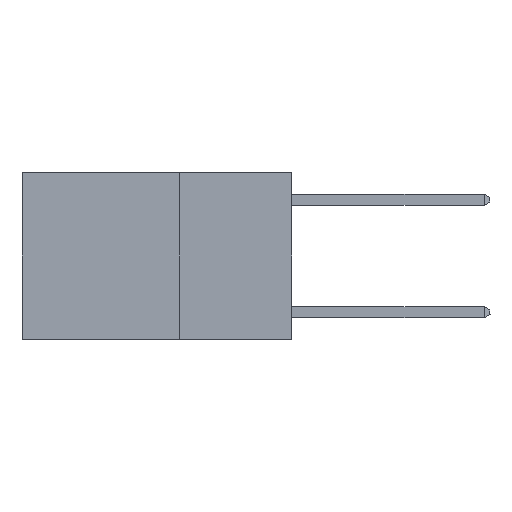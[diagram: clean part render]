
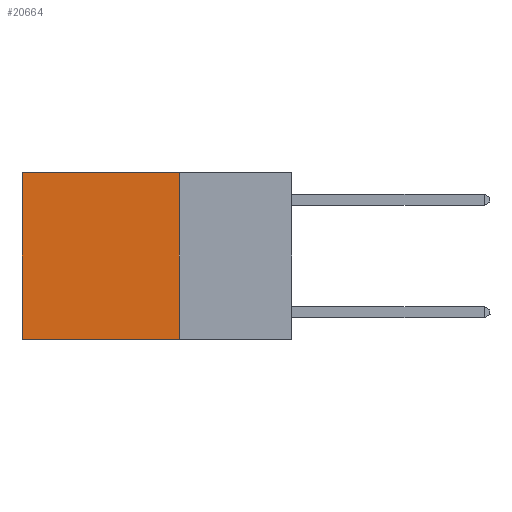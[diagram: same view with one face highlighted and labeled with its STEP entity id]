
A CAD part, left-side view. The second image highlights one B-rep face of the part: STEP entity #20664.
In plain terms, the highlighted planar face has unit normal (-1, 0, 0).
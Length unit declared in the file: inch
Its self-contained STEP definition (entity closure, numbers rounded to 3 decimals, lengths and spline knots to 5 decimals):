
#66 = CARTESIAN_POINT ( 'NONE',  ( 0.2625, 0.6, -0.37 ) ) ;
#668 = ORIENTED_EDGE ( 'NONE', *, *, #4275, .T. ) ;
#1060 = DIRECTION ( 'NONE',  ( 0., 1., 0. ) ) ;
#1570 = VECTOR ( 'NONE', #21321, 39.37008 ) ;
#3745 = VERTEX_POINT ( 'NONE', #6320 ) ;
#4275 = EDGE_CURVE ( 'NONE', #13143, #3745, #15155, .T. ) ;
#5293 = PLANE ( 'NONE',  #19595 ) ;
#5644 = LINE ( 'NONE', #13865, #16068 ) ;
#6320 = CARTESIAN_POINT ( 'NONE',  ( 0.2625, 0.6, 0. ) ) ;
#8315 = DIRECTION ( 'NONE',  ( 0., 1., 0. ) ) ;
#9969 = VERTEX_POINT ( 'NONE', #66 ) ;
#10129 = ORIENTED_EDGE ( 'NONE', *, *, #10728, .F. ) ;
#10297 = VECTOR ( 'NONE', #8315, 39.37008 ) ;
#10728 = EDGE_CURVE ( 'NONE', #13143, #25275, #23098, .T. ) ;
#11357 = ORIENTED_EDGE ( 'NONE', *, *, #24553, .T. ) ;
#11617 = DIRECTION ( 'NONE',  ( 1., 0., 0. ) ) ;
#11990 = EDGE_LOOP ( 'NONE', ( #11357, #14036, #10129, #668 ) ) ;
#13143 = VERTEX_POINT ( 'NONE', #20556 ) ;
#13865 = CARTESIAN_POINT ( 'NONE',  ( 0.2625, 0.6, 0. ) ) ;
#14036 = ORIENTED_EDGE ( 'NONE', *, *, #26895, .F. ) ;
#14658 = LINE ( 'NONE', #23928, #25558 ) ;
#15155 = LINE ( 'NONE', #18703, #10297 ) ;
#16068 = VECTOR ( 'NONE', #26135, 39.37008 ) ;
#18703 = CARTESIAN_POINT ( 'NONE',  ( 0.2625, 0.25, 0. ) ) ;
#19286 = CARTESIAN_POINT ( 'NONE',  ( 0.2625, 0.25, 0. ) ) ;
#19595 = AXIS2_PLACEMENT_3D ( 'NONE', #23962, #11617, #25987 ) ;
#19974 = FACE_OUTER_BOUND ( 'NONE', #11990, .T. ) ;
#20556 = CARTESIAN_POINT ( 'NONE',  ( 0.2625, 0.25, 0. ) ) ;
#20664 = ADVANCED_FACE ( 'NONE', ( #19974 ), #5293, .F. ) ;
#21321 = DIRECTION ( 'NONE',  ( 0., 0., -1. ) ) ;
#22459 = CARTESIAN_POINT ( 'NONE',  ( 0.2625, 0.25, -0.37 ) ) ;
#23098 = LINE ( 'NONE', #19286, #1570 ) ;
#23928 = CARTESIAN_POINT ( 'NONE',  ( 0.2625, 0.25, -0.37 ) ) ;
#23962 = CARTESIAN_POINT ( 'NONE',  ( 0.2625, 0.25, 0. ) ) ;
#24553 = EDGE_CURVE ( 'NONE', #3745, #9969, #5644, .T. ) ;
#25275 = VERTEX_POINT ( 'NONE', #22459 ) ;
#25558 = VECTOR ( 'NONE', #1060, 39.37008 ) ;
#25987 = DIRECTION ( 'NONE',  ( 0., 0., -1. ) ) ;
#26135 = DIRECTION ( 'NONE',  ( 0., 0., -1. ) ) ;
#26895 = EDGE_CURVE ( 'NONE', #25275, #9969, #14658, .T. ) ;
